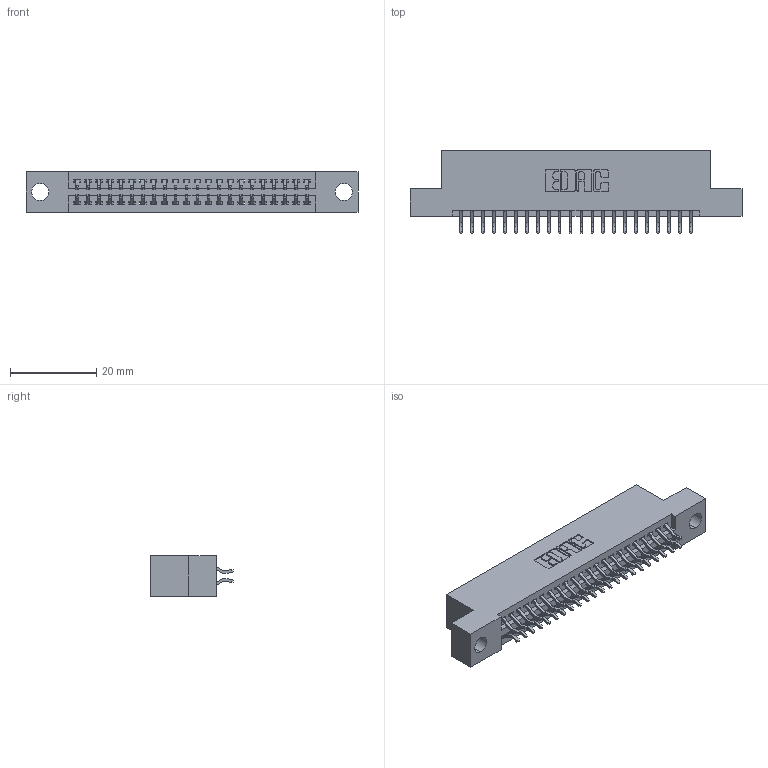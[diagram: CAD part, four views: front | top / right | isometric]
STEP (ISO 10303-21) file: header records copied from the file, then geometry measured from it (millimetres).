
FILE_DESCRIPTION (( 'STEP AP203' ), '1' );
FILE_NAME ('395-044-556-204.STEP', '2021-06-16T22:46:21', ( '' ), ( '' ), 'SwSTEP 2.0', 'SolidWorks 2020', '' );
FILE_SCHEMA (( 'CONFIG_CONTROL_DESIGN' ));
Length unit declared in the file: inch
Products named in the file (3): 345-292-001_556 Tail; 345 Part_Flush Mounting Lugs - 0.156 Dia-TI; 395-044-556-204
Assembly tree (45 placements, depth 2):
  395-044-556-204
    345 Part_Flush Mounting Lugs - 0.156 Dia-TI
    345-292-001_556 Tail  x44
Bounding box: 77.09 x 19.24 x 9.4 mm (x, y, z)
Volume: 7195.2 mm3; surface area: 10061.4 mm2
Topology: 45 solids, 45 shells, 2604 faces, 7725 edges, 5090 vertices
Faces by surface type: plane 1722, cylinder 882
Entity records: 20593 total; most frequent: CARTESIAN_POINT 3490, ORIENTED_EDGE 3410, DIRECTION 3089, EDGE_CURVE 1705, VECTOR 1477, LINE 1477, VERTEX_POINT 1134, AXIS2_PLACEMENT_3D 806
